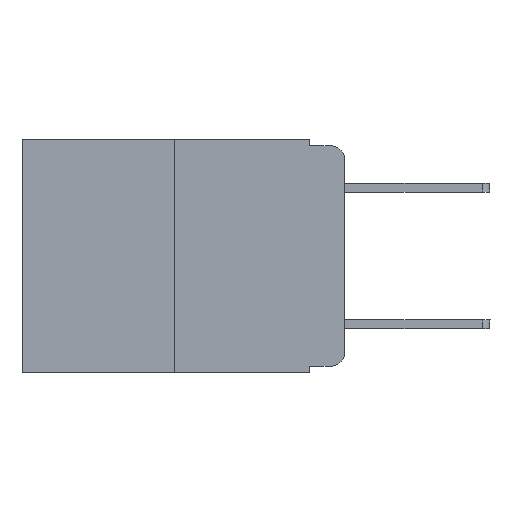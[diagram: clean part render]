
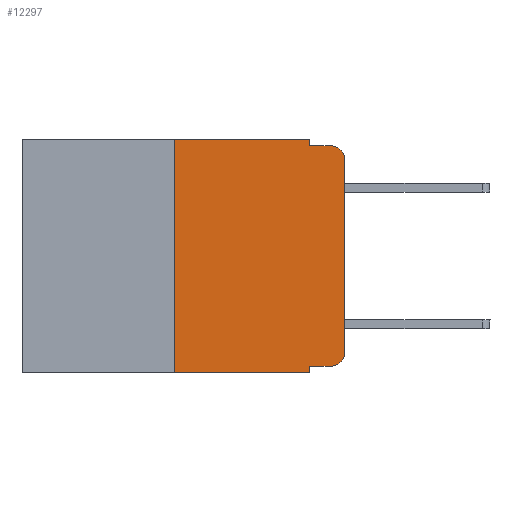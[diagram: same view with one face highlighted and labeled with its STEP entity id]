
A CAD part, left-side view. The second image highlights one B-rep face of the part: STEP entity #12297.
In plain terms, the highlighted planar face has unit normal (-1, 0, 0).
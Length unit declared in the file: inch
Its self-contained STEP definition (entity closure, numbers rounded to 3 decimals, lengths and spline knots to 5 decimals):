
#88 = EDGE_CURVE ( 'NONE', #7480, #3371, #9468, .T. ) ;
#92 = VECTOR ( 'NONE', #9996, 39.37008 ) ;
#95 = EDGE_CURVE ( 'NONE', #271, #1044, #1958, .T. ) ;
#227 = EDGE_CURVE ( 'NONE', #6285, #9074, #11977, .T. ) ;
#271 = VERTEX_POINT ( 'NONE', #8448 ) ;
#528 = VERTEX_POINT ( 'NONE', #2883 ) ;
#569 = CARTESIAN_POINT ( 'NONE',  ( 0., 0.051, -0.01 ) ) ;
#578 = LINE ( 'NONE', #8695, #10562 ) ;
#596 = ORIENTED_EDGE ( 'NONE', *, *, #88, .T. ) ;
#1022 = DIRECTION ( 'NONE',  ( -1., 0., 0. ) ) ;
#1044 = VERTEX_POINT ( 'NONE', #5052 ) ;
#1072 = CIRCLE ( 'NONE', #7258, 0.02 ) ;
#1154 = EDGE_LOOP ( 'NONE', ( #5916, #8713, #2054, #2567, #4838, #6670, #4803, #3164, #10595, #596 ) ) ;
#1479 = EDGE_CURVE ( 'NONE', #528, #6737, #2628, .T. ) ;
#1655 = DIRECTION ( 'NONE',  ( 1., 0., 0. ) ) ;
#1672 = VECTOR ( 'NONE', #7164, 39.37008 ) ;
#1958 = LINE ( 'NONE', #11061, #11386 ) ;
#2054 = ORIENTED_EDGE ( 'NONE', *, *, #227, .F. ) ;
#2218 = CARTESIAN_POINT ( 'NONE',  ( 0., 0.25, 0. ) ) ;
#2567 = ORIENTED_EDGE ( 'NONE', *, *, #10477, .F. ) ;
#2628 = LINE ( 'NONE', #5557, #7673 ) ;
#2653 = EDGE_CURVE ( 'NONE', #4085, #7480, #8705, .T. ) ;
#2829 = CARTESIAN_POINT ( 'NONE',  ( 0., 0.051, -0.01 ) ) ;
#2883 = CARTESIAN_POINT ( 'NONE',  ( 0., 0.25, -0.343 ) ) ;
#2905 = LINE ( 'NONE', #11067, #9607 ) ;
#3073 = VECTOR ( 'NONE', #10689, 39.37008 ) ;
#3157 = CARTESIAN_POINT ( 'NONE',  ( 0., 0.02, -0.03 ) ) ;
#3164 = ORIENTED_EDGE ( 'NONE', *, *, #12383, .F. ) ;
#3284 = VECTOR ( 'NONE', #6021, 39.37008 ) ;
#3351 = CARTESIAN_POINT ( 'NONE',  ( 0., 0.051, -0.333 ) ) ;
#3371 = VERTEX_POINT ( 'NONE', #10272 ) ;
#3441 = CARTESIAN_POINT ( 'NONE',  ( 0., 0.02, -0.333 ) ) ;
#3551 = DIRECTION ( 'NONE',  ( 0., -1., 0. ) ) ;
#3689 = EDGE_CURVE ( 'NONE', #3371, #9293, #2905, .T. ) ;
#3822 = DIRECTION ( 'NONE',  ( 0., -1., 0. ) ) ;
#3916 = EDGE_CURVE ( 'NONE', #9293, #9074, #1072, .T. ) ;
#4078 = CARTESIAN_POINT ( 'NONE',  ( 0., 0.051, 0. ) ) ;
#4085 = VERTEX_POINT ( 'NONE', #3351 ) ;
#4091 = DIRECTION ( 'NONE',  ( -1., 0., 0. ) ) ;
#4803 = ORIENTED_EDGE ( 'NONE', *, *, #1479, .T. ) ;
#4838 = ORIENTED_EDGE ( 'NONE', *, *, #95, .F. ) ;
#5052 = CARTESIAN_POINT ( 'NONE',  ( 0., 0.051, 0. ) ) ;
#5557 = CARTESIAN_POINT ( 'NONE',  ( 0., 0.473, -0.343 ) ) ;
#5641 = EDGE_CURVE ( 'NONE', #528, #271, #10309, .T. ) ;
#5916 = ORIENTED_EDGE ( 'NONE', *, *, #3689, .T. ) ;
#6021 = DIRECTION ( 'NONE',  ( 0., 0., -1. ) ) ;
#6285 = VERTEX_POINT ( 'NONE', #569 ) ;
#6398 = PLANE ( 'NONE',  #6704 ) ;
#6514 = CARTESIAN_POINT ( 'NONE',  ( 0., 0.051, -0.343 ) ) ;
#6605 = CARTESIAN_POINT ( 'NONE',  ( 0., 0.051, -0.333 ) ) ;
#6670 = ORIENTED_EDGE ( 'NONE', *, *, #5641, .F. ) ;
#6704 = AXIS2_PLACEMENT_3D ( 'NONE', #8817, #1655, #12950 ) ;
#6737 = VERTEX_POINT ( 'NONE', #6514 ) ;
#7164 = DIRECTION ( 'NONE',  ( 0., 0., 1. ) ) ;
#7258 = AXIS2_PLACEMENT_3D ( 'NONE', #3157, #1022, #11327 ) ;
#7480 = VERTEX_POINT ( 'NONE', #3441 ) ;
#7673 = VECTOR ( 'NONE', #3551, 39.37008 ) ;
#8234 = LINE ( 'NONE', #4078, #3284 ) ;
#8448 = CARTESIAN_POINT ( 'NONE',  ( 0., 0.25, 0. ) ) ;
#8695 = CARTESIAN_POINT ( 'NONE',  ( 0., 0.051, 0. ) ) ;
#8705 = LINE ( 'NONE', #6605, #3073 ) ;
#8713 = ORIENTED_EDGE ( 'NONE', *, *, #3916, .T. ) ;
#8816 = AXIS2_PLACEMENT_3D ( 'NONE', #11264, #4091, #9130 ) ;
#8817 = CARTESIAN_POINT ( 'NONE',  ( 0., 0.473, 0. ) ) ;
#9074 = VERTEX_POINT ( 'NONE', #12892 ) ;
#9130 = DIRECTION ( 'NONE',  ( 0., 0., -1. ) ) ;
#9293 = VERTEX_POINT ( 'NONE', #10223 ) ;
#9468 = CIRCLE ( 'NONE', #8816, 0.02 ) ;
#9607 = VECTOR ( 'NONE', #12927, 39.37008 ) ;
#9996 = DIRECTION ( 'NONE',  ( 0., -1., 0. ) ) ;
#10223 = CARTESIAN_POINT ( 'NONE',  ( 0., 0., -0.03 ) ) ;
#10272 = CARTESIAN_POINT ( 'NONE',  ( 0., 0., -0.313 ) ) ;
#10309 = LINE ( 'NONE', #2218, #1672 ) ;
#10477 = EDGE_CURVE ( 'NONE', #1044, #6285, #8234, .T. ) ;
#10562 = VECTOR ( 'NONE', #11944, 39.37008 ) ;
#10595 = ORIENTED_EDGE ( 'NONE', *, *, #2653, .T. ) ;
#10689 = DIRECTION ( 'NONE',  ( 0., -1., 0. ) ) ;
#11061 = CARTESIAN_POINT ( 'NONE',  ( 0., 0.473, 0. ) ) ;
#11067 = CARTESIAN_POINT ( 'NONE',  ( 0., 0., 0. ) ) ;
#11264 = CARTESIAN_POINT ( 'NONE',  ( 0., 0.02, -0.313 ) ) ;
#11327 = DIRECTION ( 'NONE',  ( 0., 0., -1. ) ) ;
#11386 = VECTOR ( 'NONE', #3822, 39.37008 ) ;
#11494 = FACE_OUTER_BOUND ( 'NONE', #1154, .T. ) ;
#11944 = DIRECTION ( 'NONE',  ( 0., 0., -1. ) ) ;
#11977 = LINE ( 'NONE', #2829, #92 ) ;
#12297 = ADVANCED_FACE ( 'NONE', ( #11494 ), #6398, .F. ) ;
#12383 = EDGE_CURVE ( 'NONE', #4085, #6737, #578, .T. ) ;
#12892 = CARTESIAN_POINT ( 'NONE',  ( 0., 0.02, -0.01 ) ) ;
#12927 = DIRECTION ( 'NONE',  ( 0., 0., 1. ) ) ;
#12950 = DIRECTION ( 'NONE',  ( 0., 0., -1. ) ) ;
